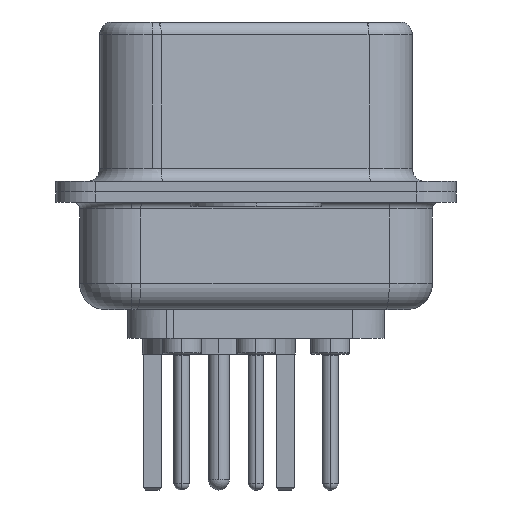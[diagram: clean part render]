
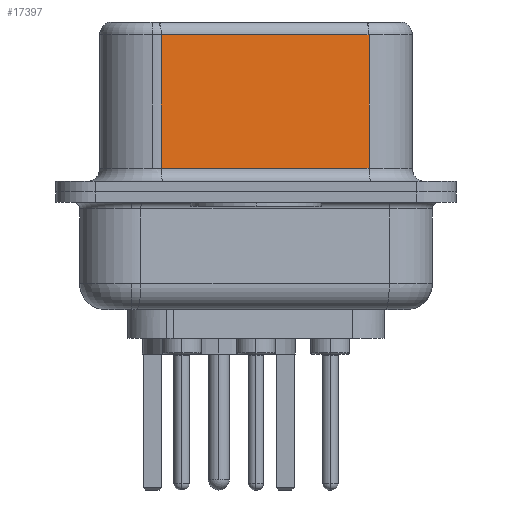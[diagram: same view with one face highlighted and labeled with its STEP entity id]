
A CAD part, left-side view. The second image highlights one B-rep face of the part: STEP entity #17397.
In plain terms, the highlighted planar face has unit normal (-0.985, -0.174, 0).
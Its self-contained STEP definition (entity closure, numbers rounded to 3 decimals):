
#1690 = DIRECTION ( 'NONE',  ( 0.985, 0.174, 0. ) ) ;
#1855 = ORIENTED_EDGE ( 'NONE', *, *, #17530, .T. ) ;
#2166 = DIRECTION ( 'NONE',  ( 0.174, -0.985, 0. ) ) ;
#2446 = EDGE_CURVE ( 'NONE', #14017, #15881, #27756, .T. ) ;
#2669 = LINE ( 'NONE', #4417, #26584 ) ;
#2795 = CARTESIAN_POINT ( 'NONE',  ( 3.73, 3.628, 6.52 ) ) ;
#3832 = ORIENTED_EDGE ( 'NONE', *, *, #2446, .F. ) ;
#4417 = CARTESIAN_POINT ( 'NONE',  ( 5.132, -4.322, 0.9 ) ) ;
#5076 = DIRECTION ( 'NONE',  ( 0., 0., -1. ) ) ;
#5753 = CARTESIAN_POINT ( 'NONE',  ( 3.73, 3.628, 0.9 ) ) ;
#5815 = CARTESIAN_POINT ( 'NONE',  ( 5.132, -4.322, 6.02 ) ) ;
#6983 = LINE ( 'NONE', #2795, #23483 ) ;
#7307 = DIRECTION ( 'NONE',  ( 0., 0., -1. ) ) ;
#9679 = VECTOR ( 'NONE', #14725, 1000. ) ;
#9847 = VECTOR ( 'NONE', #7307, 1000. ) ;
#9875 = VERTEX_POINT ( 'NONE', #11860 ) ;
#10915 = ORIENTED_EDGE ( 'NONE', *, *, #11998, .T. ) ;
#11860 = CARTESIAN_POINT ( 'NONE',  ( 3.73, 3.628, 6.02 ) ) ;
#11998 = EDGE_CURVE ( 'NONE', #9875, #23602, #6983, .T. ) ;
#13053 = ORIENTED_EDGE ( 'NONE', *, *, #19649, .T. ) ;
#14017 = VERTEX_POINT ( 'NONE', #21046 ) ;
#14725 = DIRECTION ( 'NONE',  ( -0.174, 0.985, 0. ) ) ;
#15881 = VERTEX_POINT ( 'NONE', #28252 ) ;
#17372 = DIRECTION ( 'NONE',  ( -0.174, 0.985, 0. ) ) ;
#17397 = ADVANCED_FACE ( 'NONE', ( #18832 ), #24082, .F. ) ;
#17530 = EDGE_CURVE ( 'NONE', #23602, #15881, #2669, .T. ) ;
#18832 = FACE_OUTER_BOUND ( 'NONE', #26181, .T. ) ;
#19649 = EDGE_CURVE ( 'NONE', #14017, #9875, #26860, .T. ) ;
#21046 = CARTESIAN_POINT ( 'NONE',  ( 5.132, -4.322, 6.02 ) ) ;
#22425 = AXIS2_PLACEMENT_3D ( 'NONE', #26334, #1690, #17372 ) ;
#22797 = CARTESIAN_POINT ( 'NONE',  ( 5.132, -4.322, 6.52 ) ) ;
#23483 = VECTOR ( 'NONE', #5076, 1000. ) ;
#23602 = VERTEX_POINT ( 'NONE', #5753 ) ;
#24082 = PLANE ( 'NONE',  #22425 ) ;
#26181 = EDGE_LOOP ( 'NONE', ( #3832, #13053, #10915, #1855 ) ) ;
#26334 = CARTESIAN_POINT ( 'NONE',  ( 5.132, -4.322, 6.52 ) ) ;
#26584 = VECTOR ( 'NONE', #2166, 1000. ) ;
#26860 = LINE ( 'NONE', #5815, #9679 ) ;
#27756 = LINE ( 'NONE', #22797, #9847 ) ;
#28252 = CARTESIAN_POINT ( 'NONE',  ( 5.132, -4.322, 0.9 ) ) ;
